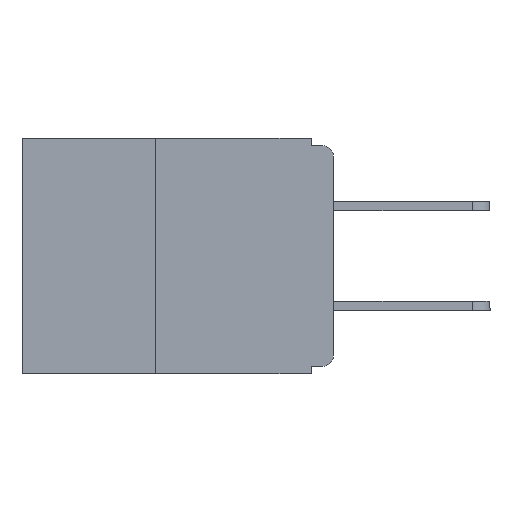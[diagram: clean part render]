
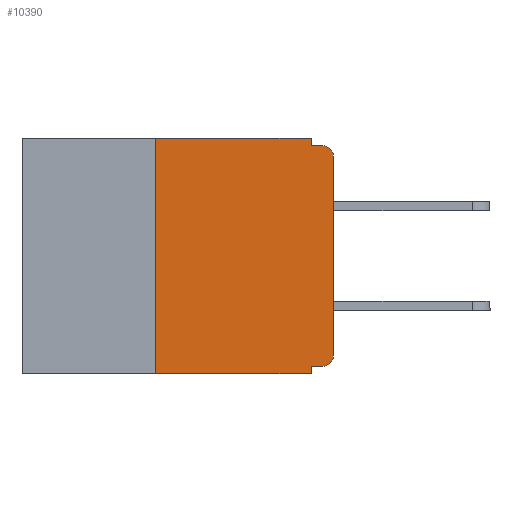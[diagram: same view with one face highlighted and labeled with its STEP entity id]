
A CAD part, left-side view. The second image highlights one B-rep face of the part: STEP entity #10390.
In plain terms, the highlighted planar face has unit normal (-1, 0, 0).
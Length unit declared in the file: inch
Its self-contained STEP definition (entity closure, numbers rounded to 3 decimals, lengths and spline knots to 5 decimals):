
#182 = VERTEX_POINT ( 'NONE', #12623 ) ;
#292 = VECTOR ( 'NONE', #5004, 39.37008 ) ;
#419 = CARTESIAN_POINT ( 'NONE',  ( 0., 0.015, -0.01 ) ) ;
#482 = ORIENTED_EDGE ( 'NONE', *, *, #10156, .F. ) ;
#892 = ORIENTED_EDGE ( 'NONE', *, *, #1875, .T. ) ;
#1010 = CARTESIAN_POINT ( 'NONE',  ( 0., 0.031, -0.33 ) ) ;
#1116 = EDGE_CURVE ( 'NONE', #10819, #8460, #1469, .T. ) ;
#1142 = CARTESIAN_POINT ( 'NONE',  ( 0., 0.015, -0.32 ) ) ;
#1221 = PLANE ( 'NONE',  #3133 ) ;
#1404 = AXIS2_PLACEMENT_3D ( 'NONE', #12852, #5108, #14098 ) ;
#1469 = LINE ( 'NONE', #12857, #7987 ) ;
#1739 = CARTESIAN_POINT ( 'NONE',  ( 0., 0., -0.32 ) ) ;
#1862 = CARTESIAN_POINT ( 'NONE',  ( 0., 0.437, -0.33 ) ) ;
#1875 = EDGE_CURVE ( 'NONE', #14991, #13005, #2596, .T. ) ;
#2309 = EDGE_CURVE ( 'NONE', #10916, #182, #12541, .T. ) ;
#2413 = ORIENTED_EDGE ( 'NONE', *, *, #15583, .F. ) ;
#2449 = DIRECTION ( 'NONE',  ( 0., 0., -1. ) ) ;
#2510 = CARTESIAN_POINT ( 'NONE',  ( 0., 0.437, 0. ) ) ;
#2596 = LINE ( 'NONE', #1862, #9147 ) ;
#2632 = EDGE_CURVE ( 'NONE', #8146, #13005, #14471, .T. ) ;
#3074 = DIRECTION ( 'NONE',  ( 0., -1., 0. ) ) ;
#3133 = AXIS2_PLACEMENT_3D ( 'NONE', #6399, #10275, #2449 ) ;
#3248 = DIRECTION ( 'NONE',  ( 0., 0., 1. ) ) ;
#4008 = DIRECTION ( 'NONE',  ( 0., -1., 0. ) ) ;
#4360 = CARTESIAN_POINT ( 'NONE',  ( 0., 0., -0.305 ) ) ;
#5004 = DIRECTION ( 'NONE',  ( 0., 0., 1. ) ) ;
#5072 = CIRCLE ( 'NONE', #13621, 0.015 ) ;
#5108 = DIRECTION ( 'NONE',  ( -1., 0., 0. ) ) ;
#5115 = CARTESIAN_POINT ( 'NONE',  ( 0., 0.25, -0.33 ) ) ;
#5325 = CARTESIAN_POINT ( 'NONE',  ( 0., 0.031, 0. ) ) ;
#6350 = DIRECTION ( 'NONE',  ( -1., 0., 0. ) ) ;
#6399 = CARTESIAN_POINT ( 'NONE',  ( 0., 0.437, 0. ) ) ;
#7174 = VERTEX_POINT ( 'NONE', #14547 ) ;
#7574 = CARTESIAN_POINT ( 'NONE',  ( 0., 0.031, -0.32 ) ) ;
#7863 = DIRECTION ( 'NONE',  ( 0., 0., -1. ) ) ;
#7876 = CARTESIAN_POINT ( 'NONE',  ( 0., 0.031, -0.33 ) ) ;
#7987 = VECTOR ( 'NONE', #4008, 39.37008 ) ;
#8146 = VERTEX_POINT ( 'NONE', #7574 ) ;
#8243 = DIRECTION ( 'NONE',  ( 0., 1., 0. ) ) ;
#8460 = VERTEX_POINT ( 'NONE', #419 ) ;
#8748 = VECTOR ( 'NONE', #8243, 39.37008 ) ;
#9131 = VECTOR ( 'NONE', #3074, 39.37008 ) ;
#9147 = VECTOR ( 'NONE', #10680, 39.37008 ) ;
#9487 = VECTOR ( 'NONE', #13076, 39.37008 ) ;
#10155 = VECTOR ( 'NONE', #3248, 39.37008 ) ;
#10156 = EDGE_CURVE ( 'NONE', #14991, #10916, #10959, .T. ) ;
#10209 = LINE ( 'NONE', #14017, #292 ) ;
#10275 = DIRECTION ( 'NONE',  ( 1., 0., 0. ) ) ;
#10344 = FACE_OUTER_BOUND ( 'NONE', #13085, .T. ) ;
#10370 = ORIENTED_EDGE ( 'NONE', *, *, #1116, .F. ) ;
#10390 = ADVANCED_FACE ( 'NONE', ( #10344 ), #1221, .F. ) ;
#10675 = VERTEX_POINT ( 'NONE', #4360 ) ;
#10680 = DIRECTION ( 'NONE',  ( 0., -1., 0. ) ) ;
#10819 = VERTEX_POINT ( 'NONE', #14938 ) ;
#10916 = VERTEX_POINT ( 'NONE', #15084 ) ;
#10959 = LINE ( 'NONE', #14846, #10155 ) ;
#11128 = VECTOR ( 'NONE', #7863, 39.37008 ) ;
#11609 = EDGE_CURVE ( 'NONE', #10675, #7174, #10209, .T. ) ;
#11904 = LINE ( 'NONE', #1739, #8748 ) ;
#12390 = VERTEX_POINT ( 'NONE', #1142 ) ;
#12487 = LINE ( 'NONE', #5325, #9487 ) ;
#12541 = LINE ( 'NONE', #2510, #9131 ) ;
#12547 = ORIENTED_EDGE ( 'NONE', *, *, #11609, .T. ) ;
#12623 = CARTESIAN_POINT ( 'NONE',  ( 0., 0.031, 0. ) ) ;
#12852 = CARTESIAN_POINT ( 'NONE',  ( 0., 0.015, -0.025 ) ) ;
#12857 = CARTESIAN_POINT ( 'NONE',  ( 0., 0., -0.01 ) ) ;
#13005 = VERTEX_POINT ( 'NONE', #1010 ) ;
#13067 = EDGE_CURVE ( 'NONE', #12390, #10675, #5072, .T. ) ;
#13076 = DIRECTION ( 'NONE',  ( 0., 0., -1. ) ) ;
#13085 = EDGE_LOOP ( 'NONE', ( #12547, #15993, #10370, #2413, #13585, #482, #892, #15670, #13983, #15483 ) ) ;
#13336 = CIRCLE ( 'NONE', #1404, 0.015 ) ;
#13585 = ORIENTED_EDGE ( 'NONE', *, *, #2309, .F. ) ;
#13619 = EDGE_CURVE ( 'NONE', #7174, #8460, #13336, .T. ) ;
#13621 = AXIS2_PLACEMENT_3D ( 'NONE', #14013, #6350, #15213 ) ;
#13882 = EDGE_CURVE ( 'NONE', #12390, #8146, #11904, .T. ) ;
#13983 = ORIENTED_EDGE ( 'NONE', *, *, #13882, .F. ) ;
#14013 = CARTESIAN_POINT ( 'NONE',  ( 0., 0.015, -0.305 ) ) ;
#14017 = CARTESIAN_POINT ( 'NONE',  ( 0., 0., 0. ) ) ;
#14098 = DIRECTION ( 'NONE',  ( 0., 0., -1. ) ) ;
#14471 = LINE ( 'NONE', #7876, #11128 ) ;
#14547 = CARTESIAN_POINT ( 'NONE',  ( 0., 0., -0.025 ) ) ;
#14846 = CARTESIAN_POINT ( 'NONE',  ( 0., 0.25, -0.33 ) ) ;
#14938 = CARTESIAN_POINT ( 'NONE',  ( 0., 0.031, -0.01 ) ) ;
#14991 = VERTEX_POINT ( 'NONE', #5115 ) ;
#15084 = CARTESIAN_POINT ( 'NONE',  ( 0., 0.25, 0. ) ) ;
#15213 = DIRECTION ( 'NONE',  ( 0., 0., -1. ) ) ;
#15483 = ORIENTED_EDGE ( 'NONE', *, *, #13067, .T. ) ;
#15583 = EDGE_CURVE ( 'NONE', #182, #10819, #12487, .T. ) ;
#15670 = ORIENTED_EDGE ( 'NONE', *, *, #2632, .F. ) ;
#15993 = ORIENTED_EDGE ( 'NONE', *, *, #13619, .T. ) ;
